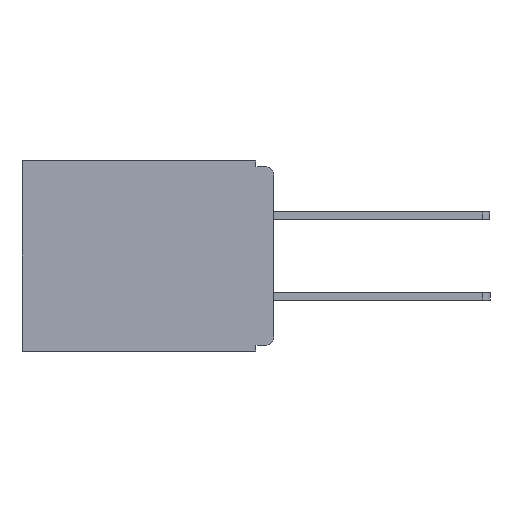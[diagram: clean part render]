
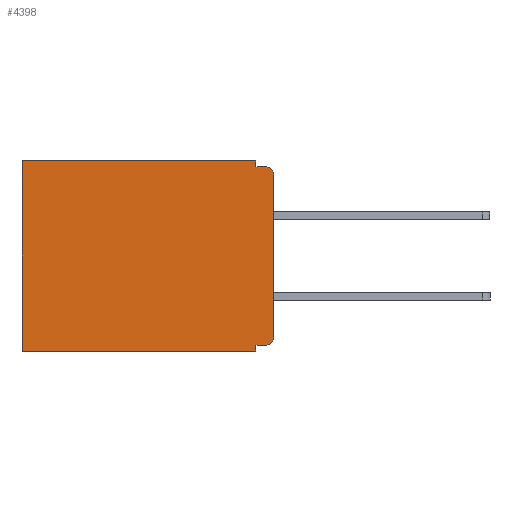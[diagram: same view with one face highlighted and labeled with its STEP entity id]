
A CAD part, left-side view. The second image highlights one B-rep face of the part: STEP entity #4398.
In plain terms, the highlighted planar face has unit normal (-1, 0, 0).
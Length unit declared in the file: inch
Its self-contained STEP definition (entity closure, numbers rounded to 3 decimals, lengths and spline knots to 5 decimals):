
#196 = VECTOR ( 'NONE', #646, 39.37008 ) ;
#646 = DIRECTION ( 'NONE',  ( 0., -1., 0. ) ) ;
#1069 = VERTEX_POINT ( 'NONE', #5992 ) ;
#1288 = VERTEX_POINT ( 'NONE', #2743 ) ;
#1381 = VERTEX_POINT ( 'NONE', #9274 ) ;
#1387 = DIRECTION ( 'NONE',  ( 0., 1., 0. ) ) ;
#1441 = CARTESIAN_POINT ( 'NONE',  ( 0.3, 0.015, -0.025 ) ) ;
#1549 = EDGE_CURVE ( 'NONE', #12669, #2487, #6872, .T. ) ;
#2067 = ORIENTED_EDGE ( 'NONE', *, *, #7662, .T. ) ;
#2074 = DIRECTION ( 'NONE',  ( 0., 0., -1. ) ) ;
#2275 = LINE ( 'NONE', #4713, #11411 ) ;
#2457 = PLANE ( 'NONE',  #15225 ) ;
#2468 = ORIENTED_EDGE ( 'NONE', *, *, #14871, .F. ) ;
#2487 = VERTEX_POINT ( 'NONE', #6658 ) ;
#2743 = CARTESIAN_POINT ( 'NONE',  ( 0.3, 0., -0.025 ) ) ;
#2758 = DIRECTION ( 'NONE',  ( 0., 0., -1. ) ) ;
#2914 = VECTOR ( 'NONE', #7927, 39.37008 ) ;
#3050 = VECTOR ( 'NONE', #8461, 39.37008 ) ;
#3159 = LINE ( 'NONE', #3937, #12211 ) ;
#3286 = FACE_OUTER_BOUND ( 'NONE', #4540, .T. ) ;
#3429 = DIRECTION ( 'NONE',  ( 0., 0., -1. ) ) ;
#3443 = CARTESIAN_POINT ( 'NONE',  ( 0.3, 0.015, -0.32 ) ) ;
#3689 = CARTESIAN_POINT ( 'NONE',  ( 0.3, 0.437, 0. ) ) ;
#3778 = DIRECTION ( 'NONE',  ( 0., 0., -1. ) ) ;
#3937 = CARTESIAN_POINT ( 'NONE',  ( 0.3, 0., 0. ) ) ;
#4032 = CARTESIAN_POINT ( 'NONE',  ( 0.3, 0.031, -0.33 ) ) ;
#4261 = EDGE_CURVE ( 'NONE', #7405, #12669, #2275, .T. ) ;
#4316 = ORIENTED_EDGE ( 'NONE', *, *, #10016, .F. ) ;
#4392 = LINE ( 'NONE', #12324, #13760 ) ;
#4398 = ADVANCED_FACE ( 'NONE', ( #3286 ), #2457, .F. ) ;
#4447 = AXIS2_PLACEMENT_3D ( 'NONE', #1441, #10179, #2758 ) ;
#4540 = EDGE_LOOP ( 'NONE', ( #14048, #5731, #2468, #4316, #6227, #2067, #7958, #9536, #8527, #5900 ) ) ;
#4713 = CARTESIAN_POINT ( 'NONE',  ( 0.3, 0.031, -0.33 ) ) ;
#4876 = AXIS2_PLACEMENT_3D ( 'NONE', #4941, #13486, #6177 ) ;
#4941 = CARTESIAN_POINT ( 'NONE',  ( 0.3, 0.015, -0.305 ) ) ;
#5570 = VERTEX_POINT ( 'NONE', #3443 ) ;
#5731 = ORIENTED_EDGE ( 'NONE', *, *, #12032, .T. ) ;
#5900 = ORIENTED_EDGE ( 'NONE', *, *, #13133, .T. ) ;
#5992 = CARTESIAN_POINT ( 'NONE',  ( 0.3, 0., -0.305 ) ) ;
#6021 = CARTESIAN_POINT ( 'NONE',  ( 0.3, 0., -0.01 ) ) ;
#6177 = DIRECTION ( 'NONE',  ( 0., 0., -1. ) ) ;
#6227 = ORIENTED_EDGE ( 'NONE', *, *, #8436, .T. ) ;
#6658 = CARTESIAN_POINT ( 'NONE',  ( 0.3, 0.437, -0.33 ) ) ;
#6872 = LINE ( 'NONE', #15858, #10112 ) ;
#7405 = VERTEX_POINT ( 'NONE', #10259 ) ;
#7452 = LINE ( 'NONE', #8317, #14337 ) ;
#7662 = EDGE_CURVE ( 'NONE', #11387, #2487, #7452, .T. ) ;
#7746 = VERTEX_POINT ( 'NONE', #12118 ) ;
#7927 = DIRECTION ( 'NONE',  ( 0., 0., -1. ) ) ;
#7958 = ORIENTED_EDGE ( 'NONE', *, *, #1549, .F. ) ;
#8317 = CARTESIAN_POINT ( 'NONE',  ( 0.3, 0.437, -0.33 ) ) ;
#8436 = EDGE_CURVE ( 'NONE', #1381, #11387, #3159, .T. ) ;
#8461 = DIRECTION ( 'NONE',  ( 0., 0., -1. ) ) ;
#8527 = ORIENTED_EDGE ( 'NONE', *, *, #11429, .F. ) ;
#9274 = CARTESIAN_POINT ( 'NONE',  ( 0.3, 0.031, 0. ) ) ;
#9536 = ORIENTED_EDGE ( 'NONE', *, *, #4261, .F. ) ;
#10016 = EDGE_CURVE ( 'NONE', #1381, #7746, #13230, .T. ) ;
#10112 = VECTOR ( 'NONE', #15285, 39.37008 ) ;
#10179 = DIRECTION ( 'NONE',  ( -1., 0., 0. ) ) ;
#10259 = CARTESIAN_POINT ( 'NONE',  ( 0.3, 0.031, -0.32 ) ) ;
#10697 = CIRCLE ( 'NONE', #4447, 0.015 ) ;
#11110 = DIRECTION ( 'NONE',  ( 0., 1., 0. ) ) ;
#11142 = DIRECTION ( 'NONE',  ( 1., 0., 0. ) ) ;
#11387 = VERTEX_POINT ( 'NONE', #3689 ) ;
#11411 = VECTOR ( 'NONE', #3429, 39.37008 ) ;
#11429 = EDGE_CURVE ( 'NONE', #5570, #7405, #4392, .T. ) ;
#12032 = EDGE_CURVE ( 'NONE', #1288, #14747, #10697, .T. ) ;
#12118 = CARTESIAN_POINT ( 'NONE',  ( 0.3, 0.031, -0.01 ) ) ;
#12211 = VECTOR ( 'NONE', #1387, 39.37008 ) ;
#12324 = CARTESIAN_POINT ( 'NONE',  ( 0.3, 0., -0.32 ) ) ;
#12669 = VERTEX_POINT ( 'NONE', #4032 ) ;
#12832 = CARTESIAN_POINT ( 'NONE',  ( 0.3, 0., -0.33 ) ) ;
#13133 = EDGE_CURVE ( 'NONE', #5570, #1069, #13700, .T. ) ;
#13230 = LINE ( 'NONE', #15742, #3050 ) ;
#13467 = EDGE_CURVE ( 'NONE', #1288, #1069, #15563, .T. ) ;
#13476 = LINE ( 'NONE', #6021, #196 ) ;
#13486 = DIRECTION ( 'NONE',  ( -1., 0., 0. ) ) ;
#13700 = CIRCLE ( 'NONE', #4876, 0.015 ) ;
#13760 = VECTOR ( 'NONE', #11110, 39.37008 ) ;
#14048 = ORIENTED_EDGE ( 'NONE', *, *, #13467, .F. ) ;
#14135 = CARTESIAN_POINT ( 'NONE',  ( 0.3, 0.015, -0.01 ) ) ;
#14337 = VECTOR ( 'NONE', #2074, 39.37008 ) ;
#14747 = VERTEX_POINT ( 'NONE', #14135 ) ;
#14871 = EDGE_CURVE ( 'NONE', #7746, #14747, #13476, .T. ) ;
#15225 = AXIS2_PLACEMENT_3D ( 'NONE', #15946, #11142, #3778 ) ;
#15285 = DIRECTION ( 'NONE',  ( 0., 1., 0. ) ) ;
#15563 = LINE ( 'NONE', #12832, #2914 ) ;
#15742 = CARTESIAN_POINT ( 'NONE',  ( 0.3, 0.031, 0. ) ) ;
#15858 = CARTESIAN_POINT ( 'NONE',  ( 0.3, 0., -0.33 ) ) ;
#15946 = CARTESIAN_POINT ( 'NONE',  ( 0.3, 0., -0.33 ) ) ;
